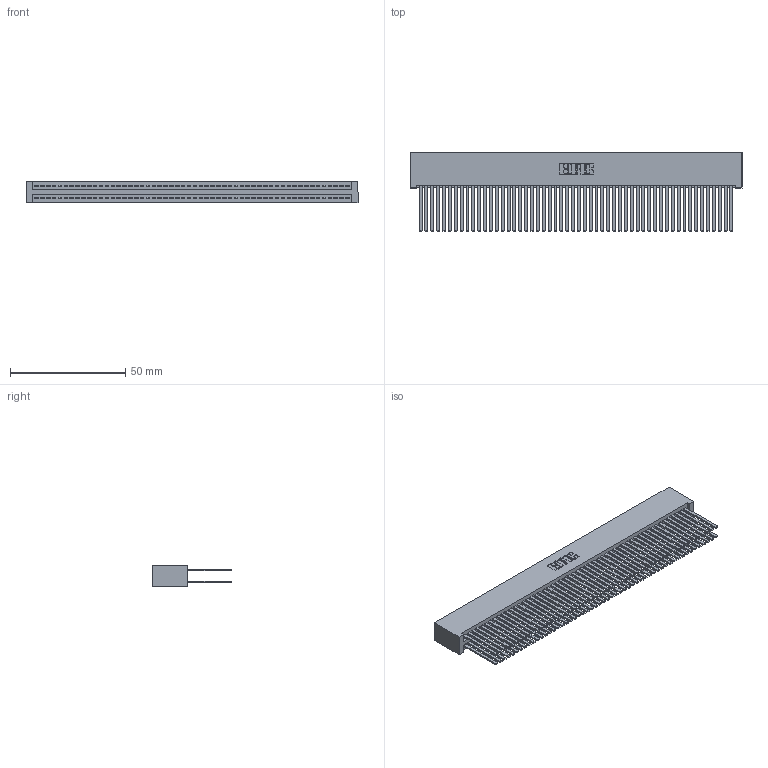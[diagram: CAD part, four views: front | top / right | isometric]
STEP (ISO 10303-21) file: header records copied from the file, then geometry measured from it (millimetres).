
FILE_DESCRIPTION (( 'STEP AP203' ), '1' );
FILE_NAME ('345-108-544-201.STEP', '2018-10-07T06:53:08', ( '' ), ( '' ), 'SwSTEP 2.0', 'SolidWorks 2016', '' );
FILE_SCHEMA (( 'CONFIG_CONTROL_DESIGN' ));
Length unit declared in the file: inch
Products named in the file (3): 345-292-001_345-293-144; 345 Part_No Mounting Lugs; 345-108-544-201
Assembly tree (109 placements, depth 2):
  345-108-544-201
    345 Part_No Mounting Lugs
    345-292-001_345-293-144  x108
Bounding box: 143.76 x 33.96 x 9.4 mm (x, y, z)
Volume: 16206.6 mm3; surface area: 28929.1 mm2
Topology: 109 solids, 109 shells, 4870 faces, 14465 edges, 9498 vertices
Faces by surface type: plane 3208, cylinder 1662
Entity records: 40293 total; most frequent: CARTESIAN_POINT 6740, ORIENTED_EDGE 6674, DIRECTION 5921, EDGE_CURVE 3337, LINE 3001, VECTOR 3001, VERTEX_POINT 2222, AXIS2_PLACEMENT_3D 1460
